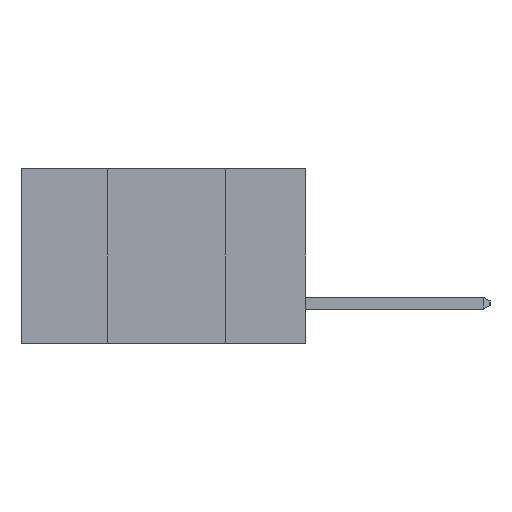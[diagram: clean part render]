
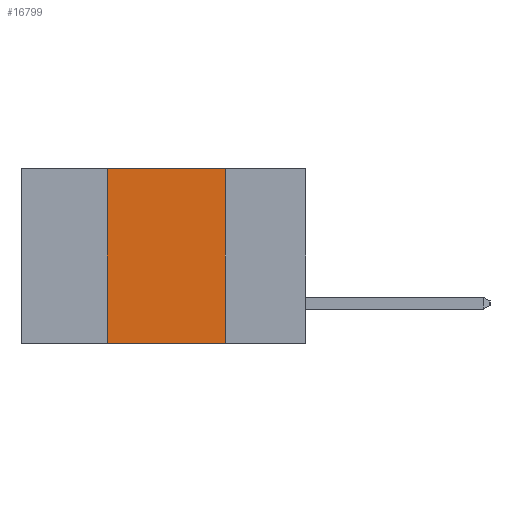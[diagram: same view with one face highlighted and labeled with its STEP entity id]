
A CAD part, left-side view. The second image highlights one B-rep face of the part: STEP entity #16799.
In plain terms, the highlighted planar face has unit normal (-1, 0, 0).
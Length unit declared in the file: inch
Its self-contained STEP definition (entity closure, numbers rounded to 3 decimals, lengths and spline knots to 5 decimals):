
#339 = CARTESIAN_POINT ( 'NONE',  ( 0., 0.17, -0.37 ) ) ;
#361 = CARTESIAN_POINT ( 'NONE',  ( 0., 0.17, 0. ) ) ;
#820 = EDGE_CURVE ( 'NONE', #8106, #9122, #8687, .T. ) ;
#1372 = VECTOR ( 'NONE', #9856, 39.37008 ) ;
#1953 = EDGE_CURVE ( 'NONE', #16201, #8106, #14542, .T. ) ;
#2299 = VERTEX_POINT ( 'NONE', #15615 ) ;
#2883 = CARTESIAN_POINT ( 'NONE',  ( 0., 0.42, 0. ) ) ;
#3305 = CARTESIAN_POINT ( 'NONE',  ( 0., 0.42, 0. ) ) ;
#4465 = VECTOR ( 'NONE', #10451, 39.37008 ) ;
#5790 = CARTESIAN_POINT ( 'NONE',  ( 0., 0.17, 0. ) ) ;
#5833 = CARTESIAN_POINT ( 'NONE',  ( 0., 0.6, 0. ) ) ;
#6635 = CARTESIAN_POINT ( 'NONE',  ( 0., 0.6, 0. ) ) ;
#6671 = DIRECTION ( 'NONE',  ( 0., -1., 0. ) ) ;
#6707 = CARTESIAN_POINT ( 'NONE',  ( 0., 0.6, -0.37 ) ) ;
#7008 = AXIS2_PLACEMENT_3D ( 'NONE', #5833, #16787, #7444 ) ;
#7444 = DIRECTION ( 'NONE',  ( 0., 0., -1. ) ) ;
#7872 = LINE ( 'NONE', #3305, #15181 ) ;
#7882 = ORIENTED_EDGE ( 'NONE', *, *, #820, .F. ) ;
#8106 = VERTEX_POINT ( 'NONE', #5790 ) ;
#8200 = EDGE_LOOP ( 'NONE', ( #7882, #20294, #12997, #17161 ) ) ;
#8687 = LINE ( 'NONE', #361, #4465 ) ;
#9122 = VERTEX_POINT ( 'NONE', #339 ) ;
#9680 = EDGE_CURVE ( 'NONE', #2299, #9122, #10716, .T. ) ;
#9856 = DIRECTION ( 'NONE',  ( 0., -1., 0. ) ) ;
#10426 = VECTOR ( 'NONE', #6671, 39.37008 ) ;
#10451 = DIRECTION ( 'NONE',  ( 0., 0., -1. ) ) ;
#10716 = LINE ( 'NONE', #6707, #1372 ) ;
#10882 = FACE_OUTER_BOUND ( 'NONE', #8200, .T. ) ;
#12636 = DIRECTION ( 'NONE',  ( 0., 0., 1. ) ) ;
#12774 = EDGE_CURVE ( 'NONE', #2299, #16201, #7872, .T. ) ;
#12997 = ORIENTED_EDGE ( 'NONE', *, *, #12774, .F. ) ;
#14542 = LINE ( 'NONE', #6635, #10426 ) ;
#15181 = VECTOR ( 'NONE', #12636, 39.37008 ) ;
#15203 = PLANE ( 'NONE',  #7008 ) ;
#15615 = CARTESIAN_POINT ( 'NONE',  ( 0., 0.42, -0.37 ) ) ;
#16201 = VERTEX_POINT ( 'NONE', #2883 ) ;
#16787 = DIRECTION ( 'NONE',  ( 1., 0., 0. ) ) ;
#16799 = ADVANCED_FACE ( 'NONE', ( #10882 ), #15203, .F. ) ;
#17161 = ORIENTED_EDGE ( 'NONE', *, *, #9680, .T. ) ;
#20294 = ORIENTED_EDGE ( 'NONE', *, *, #1953, .F. ) ;
